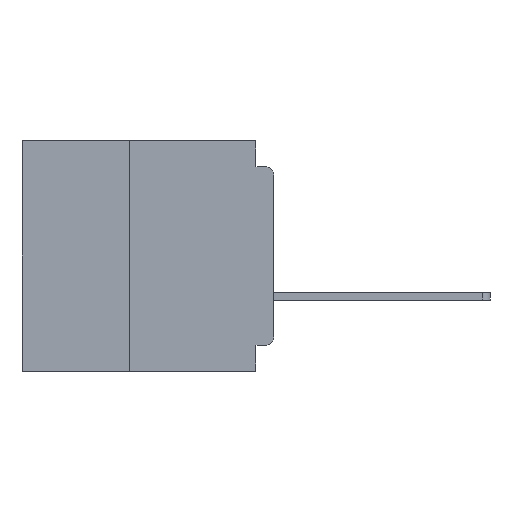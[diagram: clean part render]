
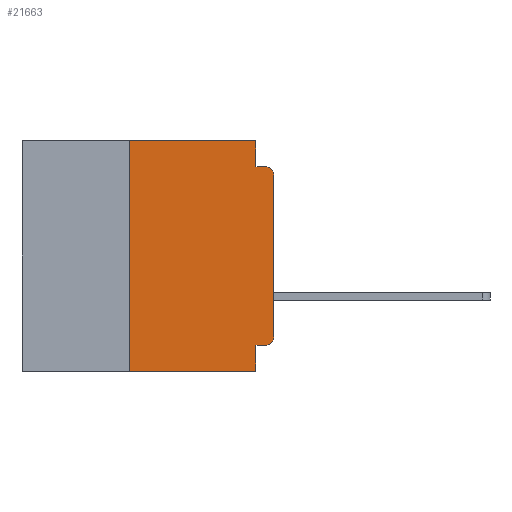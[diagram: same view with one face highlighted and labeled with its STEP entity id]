
A CAD part, left-side view. The second image highlights one B-rep face of the part: STEP entity #21663.
In plain terms, the highlighted planar face has unit normal (-1, 0, 0).
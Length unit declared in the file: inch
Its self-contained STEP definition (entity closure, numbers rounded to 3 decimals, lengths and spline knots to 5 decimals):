
#908 = PLANE ( 'NONE',  #45123 ) ;
#1219 = LINE ( 'NONE', #21102, #33795 ) ;
#2814 = ORIENTED_EDGE ( 'NONE', *, *, #13666, .F. ) ;
#4038 = DIRECTION ( 'NONE',  ( 0., 1., 0. ) ) ;
#5166 = DIRECTION ( 'NONE',  ( 0., 0., -1. ) ) ;
#6028 = CIRCLE ( 'NONE', #38460, 0.015 ) ;
#6461 = ORIENTED_EDGE ( 'NONE', *, *, #13768, .F. ) ;
#7155 = CARTESIAN_POINT ( 'NONE',  ( 0., 0.015, -0.06 ) ) ;
#7211 = ORIENTED_EDGE ( 'NONE', *, *, #46050, .F. ) ;
#7964 = VERTEX_POINT ( 'NONE', #40483 ) ;
#8088 = DIRECTION ( 'NONE',  ( -1., 0., 0. ) ) ;
#8342 = VERTEX_POINT ( 'NONE', #22267 ) ;
#9005 = VERTEX_POINT ( 'NONE', #31717 ) ;
#10769 = LINE ( 'NONE', #35894, #32813 ) ;
#11407 = DIRECTION ( 'NONE',  ( 0., 0., -1. ) ) ;
#12347 = VECTOR ( 'NONE', #34849, 39.37008 ) ;
#13403 = EDGE_CURVE ( 'NONE', #15887, #32087, #48465, .T. ) ;
#13622 = CIRCLE ( 'NONE', #45912, 0.015 ) ;
#13666 = EDGE_CURVE ( 'NONE', #35489, #39167, #1219, .T. ) ;
#13745 = ORIENTED_EDGE ( 'NONE', *, *, #29044, .F. ) ;
#13768 = EDGE_CURVE ( 'NONE', #43363, #35489, #29840, .T. ) ;
#15276 = CARTESIAN_POINT ( 'NONE',  ( 0., 0.031, 0. ) ) ;
#15466 = CARTESIAN_POINT ( 'NONE',  ( 0., 0.25, 0. ) ) ;
#15757 = EDGE_CURVE ( 'NONE', #9005, #8342, #18419, .T. ) ;
#15887 = VERTEX_POINT ( 'NONE', #53334 ) ;
#16849 = CARTESIAN_POINT ( 'NONE',  ( 0., 0., -0.355 ) ) ;
#18383 = LINE ( 'NONE', #16849, #29726 ) ;
#18419 = LINE ( 'NONE', #26991, #49672 ) ;
#20481 = ORIENTED_EDGE ( 'NONE', *, *, #34219, .T. ) ;
#20819 = CARTESIAN_POINT ( 'NONE',  ( 0., 0.031, 0. ) ) ;
#21102 = CARTESIAN_POINT ( 'NONE',  ( 0., 0.437, 0. ) ) ;
#21663 = ADVANCED_FACE ( 'NONE', ( #50947 ), #908, .F. ) ;
#22267 = CARTESIAN_POINT ( 'NONE',  ( 0., 0.015, -0.045 ) ) ;
#24574 = VERTEX_POINT ( 'NONE', #27447 ) ;
#26991 = CARTESIAN_POINT ( 'NONE',  ( 0., 0., -0.045 ) ) ;
#27294 = CARTESIAN_POINT ( 'NONE',  ( 0., 0.015, -0.355 ) ) ;
#27447 = CARTESIAN_POINT ( 'NONE',  ( 0., 0.031, -0.355 ) ) ;
#29044 = EDGE_CURVE ( 'NONE', #24574, #7964, #29053, .T. ) ;
#29053 = LINE ( 'NONE', #43400, #12347 ) ;
#29726 = VECTOR ( 'NONE', #4038, 39.37008 ) ;
#29840 = LINE ( 'NONE', #51345, #39776 ) ;
#30663 = DIRECTION ( 'NONE',  ( 1., 0., 0. ) ) ;
#31717 = CARTESIAN_POINT ( 'NONE',  ( 0., 0.031, -0.045 ) ) ;
#32087 = VERTEX_POINT ( 'NONE', #46275 ) ;
#32645 = LINE ( 'NONE', #15276, #52594 ) ;
#32813 = VECTOR ( 'NONE', #40143, 39.37008 ) ;
#33542 = CARTESIAN_POINT ( 'NONE',  ( 0., 0.015, -0.34 ) ) ;
#33795 = VECTOR ( 'NONE', #33891, 39.37008 ) ;
#33891 = DIRECTION ( 'NONE',  ( 0., -1., 0. ) ) ;
#34219 = EDGE_CURVE ( 'NONE', #43363, #7964, #10769, .T. ) ;
#34442 = DIRECTION ( 'NONE',  ( 0., 0., 1. ) ) ;
#34849 = DIRECTION ( 'NONE',  ( 0., 0., -1. ) ) ;
#35489 = VERTEX_POINT ( 'NONE', #15466 ) ;
#35894 = CARTESIAN_POINT ( 'NONE',  ( 0., 0.437, -0.4 ) ) ;
#36893 = DIRECTION ( 'NONE',  ( -1., 0., 0. ) ) ;
#37430 = EDGE_CURVE ( 'NONE', #51414, #24574, #18383, .T. ) ;
#37829 = DIRECTION ( 'NONE',  ( 0., 0., -1. ) ) ;
#37892 = ORIENTED_EDGE ( 'NONE', *, *, #13403, .T. ) ;
#37972 = EDGE_CURVE ( 'NONE', #51414, #15887, #6028, .T. ) ;
#38460 = AXIS2_PLACEMENT_3D ( 'NONE', #33542, #8088, #37829 ) ;
#38501 = VECTOR ( 'NONE', #44891, 39.37008 ) ;
#39167 = VERTEX_POINT ( 'NONE', #20819 ) ;
#39776 = VECTOR ( 'NONE', #34442, 39.37008 ) ;
#40143 = DIRECTION ( 'NONE',  ( 0., -1., 0. ) ) ;
#40483 = CARTESIAN_POINT ( 'NONE',  ( 0., 0.031, -0.4 ) ) ;
#40614 = CARTESIAN_POINT ( 'NONE',  ( 0., 0., 0. ) ) ;
#42481 = ORIENTED_EDGE ( 'NONE', *, *, #37430, .F. ) ;
#43287 = CARTESIAN_POINT ( 'NONE',  ( 0., 0.437, 0. ) ) ;
#43363 = VERTEX_POINT ( 'NONE', #50586 ) ;
#43400 = CARTESIAN_POINT ( 'NONE',  ( 0., 0.031, -0.4 ) ) ;
#44891 = DIRECTION ( 'NONE',  ( 0., 0., 1. ) ) ;
#45123 = AXIS2_PLACEMENT_3D ( 'NONE', #43287, #30663, #5166 ) ;
#45912 = AXIS2_PLACEMENT_3D ( 'NONE', #7155, #36893, #11407 ) ;
#46050 = EDGE_CURVE ( 'NONE', #39167, #9005, #32645, .T. ) ;
#46275 = CARTESIAN_POINT ( 'NONE',  ( 0., 0., -0.06 ) ) ;
#46541 = ORIENTED_EDGE ( 'NONE', *, *, #15757, .F. ) ;
#47845 = EDGE_LOOP ( 'NONE', ( #37892, #54117, #46541, #7211, #2814, #6461, #20481, #13745, #42481, #54900 ) ) ;
#48304 = DIRECTION ( 'NONE',  ( 0., -1., 0. ) ) ;
#48465 = LINE ( 'NONE', #40614, #38501 ) ;
#49672 = VECTOR ( 'NONE', #48304, 39.37008 ) ;
#50586 = CARTESIAN_POINT ( 'NONE',  ( 0., 0.25, -0.4 ) ) ;
#50947 = FACE_OUTER_BOUND ( 'NONE', #47845, .T. ) ;
#51345 = CARTESIAN_POINT ( 'NONE',  ( 0., 0.25, -0.4 ) ) ;
#51414 = VERTEX_POINT ( 'NONE', #27294 ) ;
#51583 = EDGE_CURVE ( 'NONE', #32087, #8342, #13622, .T. ) ;
#52594 = VECTOR ( 'NONE', #53423, 39.37008 ) ;
#53334 = CARTESIAN_POINT ( 'NONE',  ( 0., 0., -0.34 ) ) ;
#53423 = DIRECTION ( 'NONE',  ( 0., 0., -1. ) ) ;
#54117 = ORIENTED_EDGE ( 'NONE', *, *, #51583, .T. ) ;
#54900 = ORIENTED_EDGE ( 'NONE', *, *, #37972, .T. ) ;
